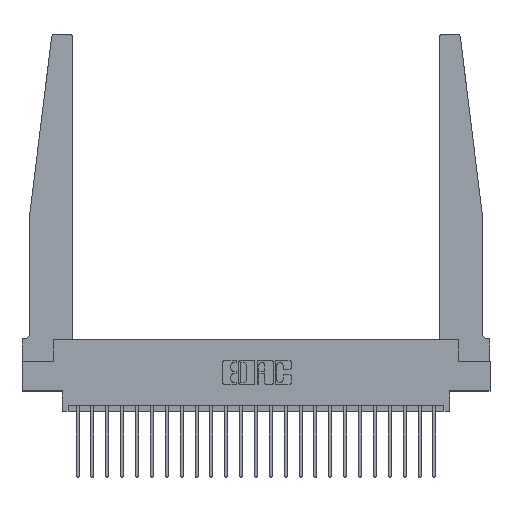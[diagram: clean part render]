
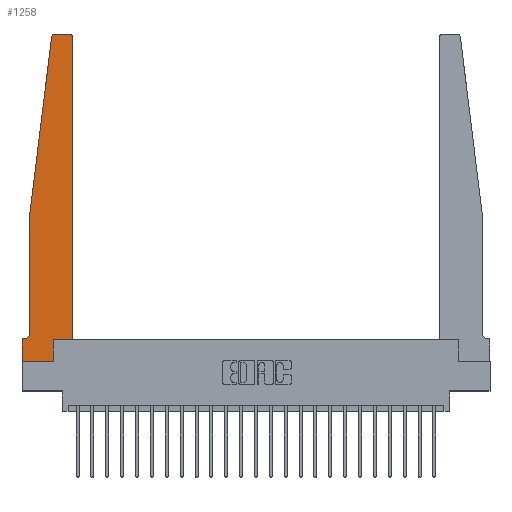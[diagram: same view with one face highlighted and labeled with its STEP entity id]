
A CAD part, top view. The second image highlights one B-rep face of the part: STEP entity #1258.
In plain terms, the highlighted planar face has unit normal (0, 0, 1).
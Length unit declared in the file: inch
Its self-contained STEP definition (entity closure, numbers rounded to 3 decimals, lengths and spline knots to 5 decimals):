
#42 = DIRECTION ( 'NONE',  ( 1., 0., 0. ) ) ;
#45 = ORIENTED_EDGE ( 'NONE', *, *, #7621, .T. ) ;
#203 = ORIENTED_EDGE ( 'NONE', *, *, #20928, .T. ) ;
#849 = DIRECTION ( 'NONE',  ( -0.122, -0.992, 0. ) ) ;
#914 = LINE ( 'NONE', #22578, #6942 ) ;
#939 = CIRCLE ( 'NONE', #3376, 0.05 ) ;
#1076 = VERTEX_POINT ( 'NONE', #19702 ) ;
#1258 = ADVANCED_FACE ( 'NONE', ( #1348 ), #20230, .T. ) ;
#1264 = DIRECTION ( 'NONE',  ( 0., 0., -1. ) ) ;
#1348 = FACE_OUTER_BOUND ( 'NONE', #9961, .T. ) ;
#1368 = ORIENTED_EDGE ( 'NONE', *, *, #4904, .T. ) ;
#1626 = DIRECTION ( 'NONE',  ( 1., 0., 0. ) ) ;
#2119 = ORIENTED_EDGE ( 'NONE', *, *, #19123, .T. ) ;
#2674 = CARTESIAN_POINT ( 'NONE',  ( 0.2605, 0., 0.37 ) ) ;
#2709 = CARTESIAN_POINT ( 'NONE',  ( 0.065, 1.25, 0.37 ) ) ;
#2805 = CARTESIAN_POINT ( 'NONE',  ( 0.425, 0.18, 0.37 ) ) ;
#2951 = AXIS2_PLACEMENT_3D ( 'NONE', #21427, #10563, #23212 ) ;
#3376 = AXIS2_PLACEMENT_3D ( 'NONE', #12228, #1264, #14087 ) ;
#3858 = CIRCLE ( 'NONE', #10137, 0.03 ) ;
#3970 = ORIENTED_EDGE ( 'NONE', *, *, #16687, .T. ) ;
#3972 = DIRECTION ( 'NONE',  ( 0., 1., 0. ) ) ;
#4603 = ORIENTED_EDGE ( 'NONE', *, *, #5684, .T. ) ;
#4620 = VECTOR ( 'NONE', #22157, 39.37008 ) ;
#4744 = ORIENTED_EDGE ( 'NONE', *, *, #15173, .T. ) ;
#4764 = VECTOR ( 'NONE', #42, 39.37008 ) ;
#4904 = EDGE_CURVE ( 'NONE', #17517, #1076, #6756, .T. ) ;
#5684 = EDGE_CURVE ( 'NONE', #18226, #14189, #10183, .T. ) ;
#5803 = VERTEX_POINT ( 'NONE', #2709 ) ;
#6112 = CARTESIAN_POINT ( 'NONE',  ( 0., 0., 0.37 ) ) ;
#6349 = ORIENTED_EDGE ( 'NONE', *, *, #21373, .T. ) ;
#6756 = LINE ( 'NONE', #8908, #15947 ) ;
#6942 = VECTOR ( 'NONE', #13554, 39.37008 ) ;
#7600 = VECTOR ( 'NONE', #3972, 39.37008 ) ;
#7621 = EDGE_CURVE ( 'NONE', #11343, #12265, #8918, .T. ) ;
#7770 = DIRECTION ( 'NONE',  ( 1., 0., 0. ) ) ;
#7969 = DIRECTION ( 'NONE',  ( 0., -1., 0. ) ) ;
#8025 = CARTESIAN_POINT ( 'NONE',  ( 0.065, 0.1875, 0.37 ) ) ;
#8521 = VECTOR ( 'NONE', #7969, 39.37008 ) ;
#8908 = CARTESIAN_POINT ( 'NONE',  ( 0.25, 2.75, 0.37 ) ) ;
#8918 = LINE ( 'NONE', #8025, #4620 ) ;
#9125 = VERTEX_POINT ( 'NONE', #12476 ) ;
#9311 = CARTESIAN_POINT ( 'NONE',  ( 0., 0.1875, 0.37 ) ) ;
#9649 = LINE ( 'NONE', #21865, #4764 ) ;
#9770 = ORIENTED_EDGE ( 'NONE', *, *, #17177, .T. ) ;
#9782 = VERTEX_POINT ( 'NONE', #21441 ) ;
#9961 = EDGE_LOOP ( 'NONE', ( #1368, #2119, #4744, #9770, #3970, #45, #203, #4603, #17772, #6349, #19094, #15940 ) ) ;
#10010 = CARTESIAN_POINT ( 'NONE',  ( 0.065, 1.25, 0.37 ) ) ;
#10137 = AXIS2_PLACEMENT_3D ( 'NONE', #23430, #12578, #1626 ) ;
#10183 = LINE ( 'NONE', #18790, #19315 ) ;
#10563 = DIRECTION ( 'NONE',  ( 0., 0., 1. ) ) ;
#10766 = VERTEX_POINT ( 'NONE', #22487 ) ;
#11146 = DIRECTION ( 'NONE',  ( 1., 0., 0. ) ) ;
#11179 = EDGE_CURVE ( 'NONE', #14189, #9782, #14920, .T. ) ;
#11264 = CARTESIAN_POINT ( 'NONE',  ( 0.425, 0.18, 0.37 ) ) ;
#11343 = VERTEX_POINT ( 'NONE', #22919 ) ;
#11602 = CARTESIAN_POINT ( 'NONE',  ( 0.2605, 0.18, 0.37 ) ) ;
#12151 = VERTEX_POINT ( 'NONE', #13401 ) ;
#12228 = CARTESIAN_POINT ( 'NONE',  ( 0.015, 0.2375, 0.37 ) ) ;
#12265 = VERTEX_POINT ( 'NONE', #15610 ) ;
#12476 = CARTESIAN_POINT ( 'NONE',  ( 0.065, 0.2375, 0.37 ) ) ;
#12555 = DIRECTION ( 'NONE',  ( -1., 0., 0. ) ) ;
#12578 = DIRECTION ( 'NONE',  ( 0., 0., 1. ) ) ;
#13186 = CARTESIAN_POINT ( 'NONE',  ( 0., 0., 0.37 ) ) ;
#13401 = CARTESIAN_POINT ( 'NONE',  ( 0.24675, 2.72367, 0.37 ) ) ;
#13554 = DIRECTION ( 'NONE',  ( 0., -1., 0. ) ) ;
#14087 = DIRECTION ( 'NONE',  ( -1., 0., 0. ) ) ;
#14189 = VERTEX_POINT ( 'NONE', #2674 ) ;
#14920 = LINE ( 'NONE', #11602, #19762 ) ;
#14988 = EDGE_CURVE ( 'NONE', #21741, #10766, #21559, .T. ) ;
#15173 = EDGE_CURVE ( 'NONE', #12151, #5803, #18184, .T. ) ;
#15459 = EDGE_CURVE ( 'NONE', #10766, #17517, #3858, .T. ) ;
#15610 = CARTESIAN_POINT ( 'NONE',  ( 0., 0.1875, 0.37 ) ) ;
#15940 = ORIENTED_EDGE ( 'NONE', *, *, #15459, .T. ) ;
#15947 = VECTOR ( 'NONE', #12555, 39.37008 ) ;
#16553 = CARTESIAN_POINT ( 'NONE',  ( 0.395, 2.75, 0.37 ) ) ;
#16687 = EDGE_CURVE ( 'NONE', #9125, #11343, #939, .T. ) ;
#16870 = CIRCLE ( 'NONE', #2951, 0.03 ) ;
#17177 = EDGE_CURVE ( 'NONE', #5803, #9125, #914, .T. ) ;
#17517 = VERTEX_POINT ( 'NONE', #16553 ) ;
#17627 = VECTOR ( 'NONE', #849, 39.37008 ) ;
#17763 = AXIS2_PLACEMENT_3D ( 'NONE', #9311, #22006, #11146 ) ;
#17772 = ORIENTED_EDGE ( 'NONE', *, *, #11179, .T. ) ;
#18184 = LINE ( 'NONE', #10010, #17627 ) ;
#18226 = VERTEX_POINT ( 'NONE', #13186 ) ;
#18790 = CARTESIAN_POINT ( 'NONE',  ( 0., 0., 0.37 ) ) ;
#19094 = ORIENTED_EDGE ( 'NONE', *, *, #14988, .T. ) ;
#19123 = EDGE_CURVE ( 'NONE', #1076, #12151, #16870, .T. ) ;
#19315 = VECTOR ( 'NONE', #7770, 39.37008 ) ;
#19702 = CARTESIAN_POINT ( 'NONE',  ( 0.27653, 2.75, 0.37 ) ) ;
#19762 = VECTOR ( 'NONE', #22534, 39.37008 ) ;
#20230 = PLANE ( 'NONE',  #17763 ) ;
#20928 = EDGE_CURVE ( 'NONE', #12265, #18226, #22983, .T. ) ;
#21373 = EDGE_CURVE ( 'NONE', #9782, #21741, #9649, .T. ) ;
#21427 = CARTESIAN_POINT ( 'NONE',  ( 0.27653, 2.72, 0.37 ) ) ;
#21441 = CARTESIAN_POINT ( 'NONE',  ( 0.2605, 0.18, 0.37 ) ) ;
#21559 = LINE ( 'NONE', #11264, #7600 ) ;
#21741 = VERTEX_POINT ( 'NONE', #2805 ) ;
#21865 = CARTESIAN_POINT ( 'NONE',  ( 0.425, 0.18, 0.37 ) ) ;
#22006 = DIRECTION ( 'NONE',  ( 0., 0., 1. ) ) ;
#22157 = DIRECTION ( 'NONE',  ( -1., 0., 0. ) ) ;
#22487 = CARTESIAN_POINT ( 'NONE',  ( 0.425, 2.72, 0.37 ) ) ;
#22534 = DIRECTION ( 'NONE',  ( 0., 1., 0. ) ) ;
#22578 = CARTESIAN_POINT ( 'NONE',  ( 0.065, 1.25, 0.37 ) ) ;
#22919 = CARTESIAN_POINT ( 'NONE',  ( 0.015, 0.1875, 0.37 ) ) ;
#22983 = LINE ( 'NONE', #6112, #8521 ) ;
#23212 = DIRECTION ( 'NONE',  ( 1., 0., 0. ) ) ;
#23430 = CARTESIAN_POINT ( 'NONE',  ( 0.395, 2.72, 0.37 ) ) ;
